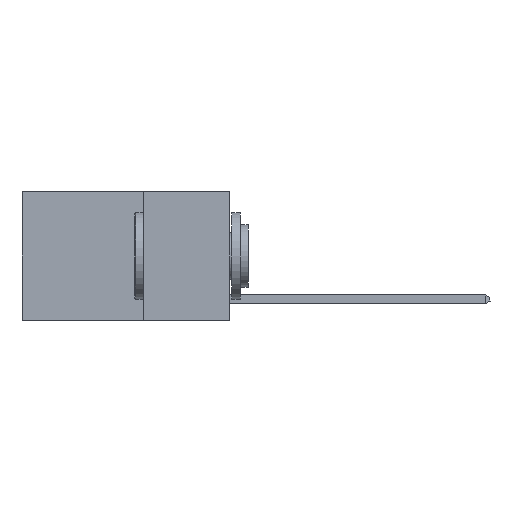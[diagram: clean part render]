
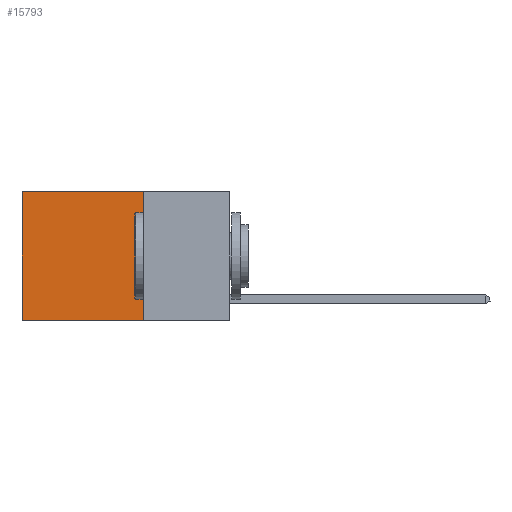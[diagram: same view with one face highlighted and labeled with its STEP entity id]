
A CAD part, left-side view. The second image highlights one B-rep face of the part: STEP entity #15793.
In plain terms, the highlighted planar face has unit normal (-1, 0, 0).
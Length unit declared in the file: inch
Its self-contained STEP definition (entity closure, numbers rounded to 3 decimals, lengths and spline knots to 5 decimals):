
#209 = VERTEX_POINT ( 'NONE', #16789 ) ;
#307 = FACE_OUTER_BOUND ( 'NONE', #7794, .T. ) ;
#412 = DIRECTION ( 'NONE',  ( 0., 0., -1. ) ) ;
#990 = VERTEX_POINT ( 'NONE', #16465 ) ;
#1175 = ORIENTED_EDGE ( 'NONE', *, *, #10488, .T. ) ;
#1680 = VERTEX_POINT ( 'NONE', #6899 ) ;
#1712 = LINE ( 'NONE', #3085, #15085 ) ;
#1767 = DIRECTION ( 'NONE',  ( 0., 1., 0. ) ) ;
#2018 = ORIENTED_EDGE ( 'NONE', *, *, #18058, .T. ) ;
#2212 = VECTOR ( 'NONE', #1767, 39.37008 ) ;
#2508 = VECTOR ( 'NONE', #412, 39.37008 ) ;
#3085 = CARTESIAN_POINT ( 'NONE',  ( 0.2625, 0.6, 0. ) ) ;
#3146 = CARTESIAN_POINT ( 'NONE',  ( 0.2625, 0.25, 0. ) ) ;
#3442 = LINE ( 'NONE', #6169, #2508 ) ;
#4794 = ORIENTED_EDGE ( 'NONE', *, *, #15734, .F. ) ;
#5288 = CARTESIAN_POINT ( 'NONE',  ( 0.2625, 0.25, 0. ) ) ;
#5396 = CARTESIAN_POINT ( 'NONE',  ( 0.2625, 0.25, -0.37 ) ) ;
#5745 = VECTOR ( 'NONE', #14119, 39.37008 ) ;
#6169 = CARTESIAN_POINT ( 'NONE',  ( 0.2625, 0.25, 0. ) ) ;
#6899 = CARTESIAN_POINT ( 'NONE',  ( 0.2625, 0.6, 0. ) ) ;
#7705 = DIRECTION ( 'NONE',  ( 0., 0., -1. ) ) ;
#7794 = EDGE_LOOP ( 'NONE', ( #2018, #9378, #4794, #1175 ) ) ;
#9129 = DIRECTION ( 'NONE',  ( 1., 0., 0. ) ) ;
#9244 = VERTEX_POINT ( 'NONE', #5288 ) ;
#9378 = ORIENTED_EDGE ( 'NONE', *, *, #10603, .F. ) ;
#10488 = EDGE_CURVE ( 'NONE', #9244, #1680, #18157, .T. ) ;
#10603 = EDGE_CURVE ( 'NONE', #209, #990, #12755, .T. ) ;
#10607 = PLANE ( 'NONE',  #16303 ) ;
#12755 = LINE ( 'NONE', #5396, #5745 ) ;
#13634 = DIRECTION ( 'NONE',  ( 0., 0., -1. ) ) ;
#14119 = DIRECTION ( 'NONE',  ( 0., 1., 0. ) ) ;
#15085 = VECTOR ( 'NONE', #7705, 39.37008 ) ;
#15734 = EDGE_CURVE ( 'NONE', #9244, #209, #3442, .T. ) ;
#15793 = ADVANCED_FACE ( 'NONE', ( #307 ), #10607, .F. ) ;
#16303 = AXIS2_PLACEMENT_3D ( 'NONE', #3146, #9129, #13634 ) ;
#16465 = CARTESIAN_POINT ( 'NONE',  ( 0.2625, 0.6, -0.37 ) ) ;
#16695 = CARTESIAN_POINT ( 'NONE',  ( 0.2625, 0.25, 0. ) ) ;
#16789 = CARTESIAN_POINT ( 'NONE',  ( 0.2625, 0.25, -0.37 ) ) ;
#18058 = EDGE_CURVE ( 'NONE', #1680, #990, #1712, .T. ) ;
#18157 = LINE ( 'NONE', #16695, #2212 ) ;
